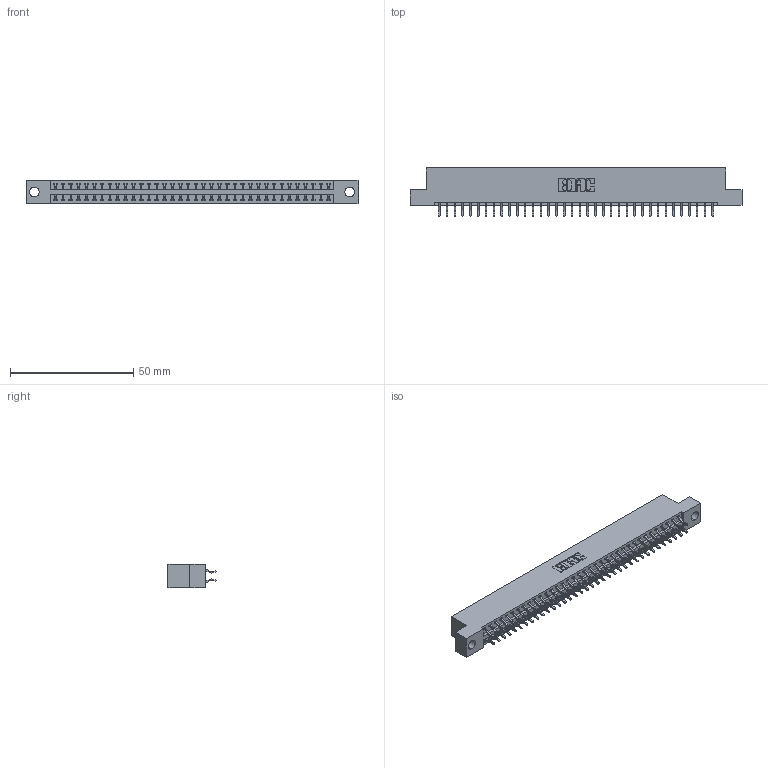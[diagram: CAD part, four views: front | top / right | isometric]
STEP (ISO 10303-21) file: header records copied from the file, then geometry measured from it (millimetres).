
FILE_DESCRIPTION (( 'STEP AP203' ), '1' );
FILE_NAME ('346-072-556-204.STEP', '2022-05-25T00:33:04', ( '' ), ( '' ), 'SwSTEP 2.0', 'SolidWorks 2020', '' );
FILE_SCHEMA (( 'CONFIG_CONTROL_DESIGN' ));
Length unit declared in the file: inch
Products named in the file (3): 346 Part_Flush Mounting Lugs - 0.156 Dia-TH; 346-072-556-204; 345-292-001_556 Tail
Assembly tree (73 placements, depth 2):
  346-072-556-204
    346 Part_Flush Mounting Lugs - 0.156 Dia-TH
    345-292-001_556 Tail  x72
Bounding box: 134.87 x 19.57 x 9.4 mm (x, y, z)
Volume: 12996.5 mm3; surface area: 17551.2 mm2
Topology: 73 solids, 73 shells, 4312 faces, 12821 edges, 8450 vertices
Faces by surface type: plane 2898, cylinder 1414
Entity records: 24941 total; most frequent: CARTESIAN_POINT 4138, ORIENTED_EDGE 4058, DIRECTION 3685, EDGE_CURVE 2029, LINE 1745, VECTOR 1745, VERTEX_POINT 1350, AXIS2_PLACEMENT_3D 970
